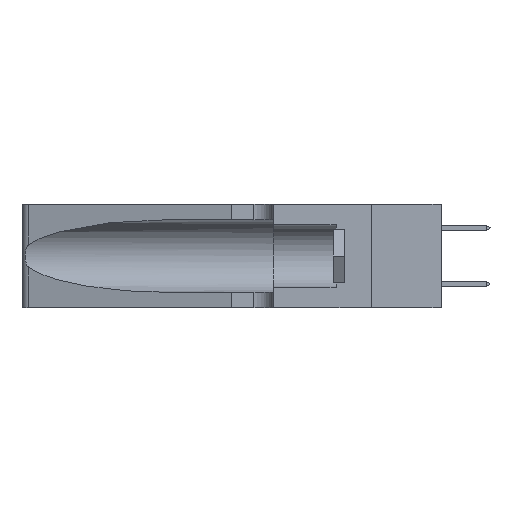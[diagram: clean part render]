
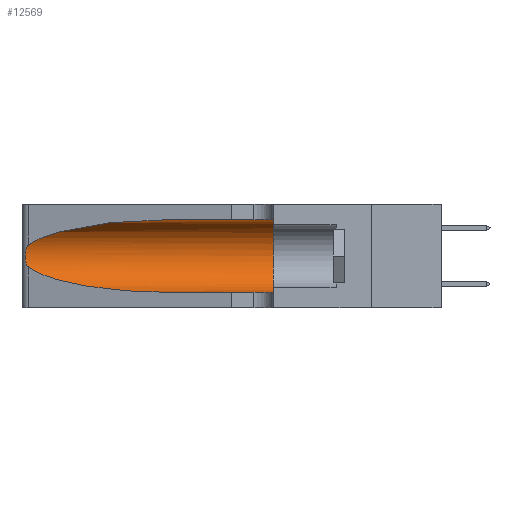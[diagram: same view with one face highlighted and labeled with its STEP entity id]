
A CAD part, left-side view. The second image highlights one B-rep face of the part: STEP entity #12569.
In plain terms, the highlighted cylindrical face has radius 3.308 mm (diameter 6.617 mm), a partial arc.
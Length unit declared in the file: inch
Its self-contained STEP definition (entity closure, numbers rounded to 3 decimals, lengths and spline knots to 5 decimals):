
#459 = DIRECTION ( 'NONE',  ( 0., -1., 0. ) ) ;
#744 = CARTESIAN_POINT ( 'NONE',  ( 0.25487, 1.22718, 0.14631 ) ) ;
#781 = DIRECTION ( 'NONE',  ( 0., -1., 0. ) ) ;
#1372 =( BOUNDED_CURVE ( )  B_SPLINE_CURVE ( 3, ( #1820, #15467, #6380, #22034 ),
 .UNSPECIFIED., .F., .F. ) 
 B_SPLINE_CURVE_WITH_KNOTS ( ( 4, 4 ),
 ( 1.5708, 2.84003 ),
 .UNSPECIFIED. ) 
 CURVE ( )  GEOMETRIC_REPRESENTATION_ITEM ( )  RATIONAL_B_SPLINE_CURVE ( ( 1., 0.87, 0.87, 1. ) ) 
 REPRESENTATION_ITEM ( '' )  );
#1820 = CARTESIAN_POINT ( 'NONE',  ( 0.1305, 0.72297, 0.31525 ) ) ;
#2820 = EDGE_CURVE ( 'NONE', #28287, #7098, #9654, .T. ) ;
#2915 = CARTESIAN_POINT ( 'NONE',  ( 0.25639, 1.23184, 0.21858 ) ) ;
#3031 = DIRECTION ( 'NONE',  ( 0., -1., 0. ) ) ;
#3348 = CARTESIAN_POINT ( 'NONE',  ( 0.1305, 0.35, 0.185 ) ) ;
#3354 = CARTESIAN_POINT ( 'NONE',  ( 0.1305, 0.35, 0.05475 ) ) ;
#4090 = AXIS2_PLACEMENT_3D ( 'NONE', #9869, #781, #23116 ) ;
#4109 = ORIENTED_EDGE ( 'NONE', *, *, #12648, .F. ) ;
#4449 = B_SPLINE_CURVE_WITH_KNOTS ( 'NONE', 3,
 ( #25125, #9730, #2915, #18702, #5172, #20867, #7480, #23077, #9828, #25217, #12128, #27378, #14419, #744 ),
 .UNSPECIFIED., .F., .F.,
 ( 4, 2, 2, 2, 2, 2, 4 ),
 ( 0., 0.00027, 0.00053, 0.00107, 0.0016, 0.00187, 0.00214 ),
 .UNSPECIFIED. ) ;
#4653 = VERTEX_POINT ( 'NONE', #18666 ) ;
#5172 = CARTESIAN_POINT ( 'NONE',  ( 0.25854, 1.2359, 0.20912 ) ) ;
#5621 = DIRECTION ( 'NONE',  ( 0., 0., 1. ) ) ;
#5741 = ORIENTED_EDGE ( 'NONE', *, *, #10207, .T. ) ;
#6133 = CARTESIAN_POINT ( 'NONE',  ( 0.1305, 0.72297, 0.05475 ) ) ;
#6211 = CIRCLE ( 'NONE', #10285, 0.13025 ) ;
#6380 = CARTESIAN_POINT ( 'NONE',  ( 0.2373, 1.15595, 0.28018 ) ) ;
#6427 = EDGE_LOOP ( 'NONE', ( #11662, #28492, #5741, #10350, #4109, #26847 ) ) ;
#7098 = VERTEX_POINT ( 'NONE', #3354 ) ;
#7480 = CARTESIAN_POINT ( 'NONE',  ( 0.26075, 1.23896, 0.19203 ) ) ;
#7657 = CYLINDRICAL_SURFACE ( 'NONE', #4090, 0.13025 ) ;
#8393 = FACE_OUTER_BOUND ( 'NONE', #6427, .T. ) ;
#8627 = VERTEX_POINT ( 'NONE', #15817 ) ;
#9654 = LINE ( 'NONE', #27105, #25836 ) ;
#9730 = CARTESIAN_POINT ( 'NONE',  ( 0.25555, 1.22994, 0.2215 ) ) ;
#9828 = CARTESIAN_POINT ( 'NONE',  ( 0.26017, 1.23833, 0.17102 ) ) ;
#9869 = CARTESIAN_POINT ( 'NONE',  ( 0.1305, 1.61858, 0.185 ) ) ;
#10207 = EDGE_CURVE ( 'NONE', #4653, #28287, #17198, .T. ) ;
#10285 = AXIS2_PLACEMENT_3D ( 'NONE', #3348, #19117, #5621 ) ;
#10350 = ORIENTED_EDGE ( 'NONE', *, *, #2820, .T. ) ;
#10693 = CARTESIAN_POINT ( 'NONE',  ( 0.2373, 1.15595, 0.08982 ) ) ;
#11662 = ORIENTED_EDGE ( 'NONE', *, *, #17620, .T. ) ;
#12128 = CARTESIAN_POINT ( 'NONE',  ( 0.25789, 1.23486, 0.15765 ) ) ;
#12569 = ADVANCED_FACE ( 'NONE', ( #8393 ), #7657, .F. ) ;
#12648 = EDGE_CURVE ( 'NONE', #16061, #7098, #6211, .T. ) ;
#14419 = CARTESIAN_POINT ( 'NONE',  ( 0.25555, 1.22993, 0.14849 ) ) ;
#14748 = LINE ( 'NONE', #20980, #26272 ) ;
#15467 = CARTESIAN_POINT ( 'NONE',  ( 0.18966, 0.96281, 0.31525 ) ) ;
#15817 = CARTESIAN_POINT ( 'NONE',  ( 0.25487, 1.22718, 0.22369 ) ) ;
#16061 = VERTEX_POINT ( 'NONE', #25600 ) ;
#17198 =( BOUNDED_CURVE ( )  B_SPLINE_CURVE ( 3, ( #26039, #10693, #19614, #6133 ),
 .UNSPECIFIED., .F., .T. ) 
 B_SPLINE_CURVE_WITH_KNOTS ( ( 4, 4 ),
 ( 3.44316, 4.71239 ),
 .UNSPECIFIED. ) 
 CURVE ( )  GEOMETRIC_REPRESENTATION_ITEM ( )  RATIONAL_B_SPLINE_CURVE ( ( 1., 0.87, 0.87, 1. ) ) 
 REPRESENTATION_ITEM ( '' )  );
#17620 = EDGE_CURVE ( 'NONE', #25923, #8627, #1372, .T. ) ;
#18666 = CARTESIAN_POINT ( 'NONE',  ( 0.25487, 1.22718, 0.14631 ) ) ;
#18702 = CARTESIAN_POINT ( 'NONE',  ( 0.25787, 1.23484, 0.2124 ) ) ;
#19117 = DIRECTION ( 'NONE',  ( 0., 1., 0. ) ) ;
#19614 = CARTESIAN_POINT ( 'NONE',  ( 0.18966, 0.96281, 0.05475 ) ) ;
#19801 = CARTESIAN_POINT ( 'NONE',  ( 0.1305, 0.72297, 0.31525 ) ) ;
#20867 = CARTESIAN_POINT ( 'NONE',  ( 0.26018, 1.23835, 0.19895 ) ) ;
#20980 = CARTESIAN_POINT ( 'NONE',  ( 0.1305, 1.61858, 0.31525 ) ) ;
#22034 = CARTESIAN_POINT ( 'NONE',  ( 0.25487, 1.22718, 0.22369 ) ) ;
#23077 = CARTESIAN_POINT ( 'NONE',  ( 0.26075, 1.23896, 0.178 ) ) ;
#23116 = DIRECTION ( 'NONE',  ( 0., 0., -1. ) ) ;
#24298 = CARTESIAN_POINT ( 'NONE',  ( 0.1305, 0.72297, 0.05475 ) ) ;
#24710 = EDGE_CURVE ( 'NONE', #8627, #4653, #4449, .T. ) ;
#25125 = CARTESIAN_POINT ( 'NONE',  ( 0.25487, 1.22718, 0.22369 ) ) ;
#25217 = CARTESIAN_POINT ( 'NONE',  ( 0.25856, 1.23593, 0.16098 ) ) ;
#25600 = CARTESIAN_POINT ( 'NONE',  ( 0.1305, 0.35, 0.31525 ) ) ;
#25836 = VECTOR ( 'NONE', #459, 39.37008 ) ;
#25923 = VERTEX_POINT ( 'NONE', #19801 ) ;
#26039 = CARTESIAN_POINT ( 'NONE',  ( 0.25487, 1.22718, 0.14631 ) ) ;
#26272 = VECTOR ( 'NONE', #3031, 39.37008 ) ;
#26847 = ORIENTED_EDGE ( 'NONE', *, *, #27913, .F. ) ;
#27105 = CARTESIAN_POINT ( 'NONE',  ( 0.1305, 1.61858, 0.05475 ) ) ;
#27378 = CARTESIAN_POINT ( 'NONE',  ( 0.25639, 1.23186, 0.15144 ) ) ;
#27913 = EDGE_CURVE ( 'NONE', #25923, #16061, #14748, .T. ) ;
#28287 = VERTEX_POINT ( 'NONE', #24298 ) ;
#28492 = ORIENTED_EDGE ( 'NONE', *, *, #24710, .T. ) ;
